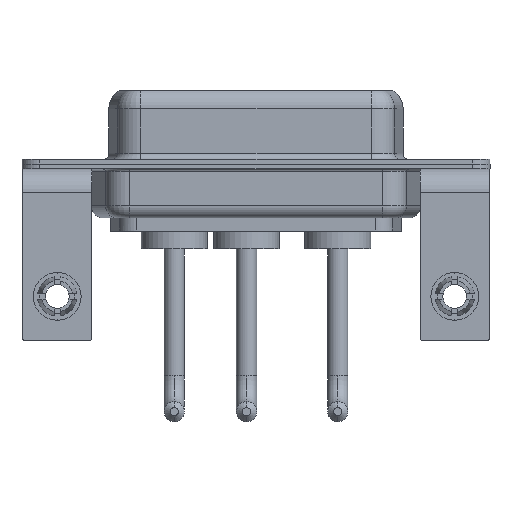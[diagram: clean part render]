
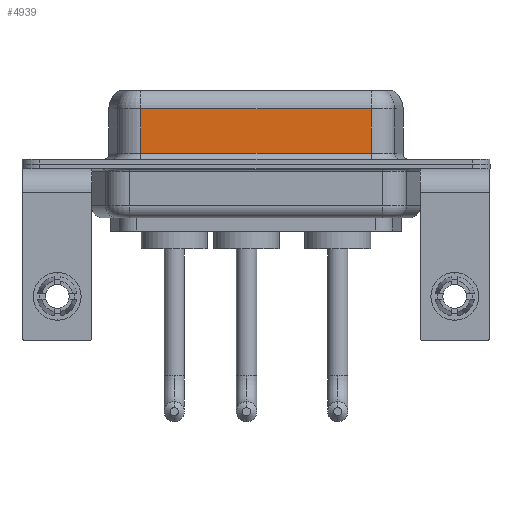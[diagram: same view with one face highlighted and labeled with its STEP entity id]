
A CAD part, front view. The second image highlights one B-rep face of the part: STEP entity #4939.
In plain terms, the highlighted planar face has unit normal (0, -1, 0).
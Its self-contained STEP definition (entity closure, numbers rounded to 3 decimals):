
#678 = DIRECTION ( 'NONE',  ( -1., 0., 0. ) ) ;
#1206 = DIRECTION ( 'NONE',  ( 0., 0., 1. ) ) ;
#1521 = ORIENTED_EDGE ( 'NONE', *, *, #10036, .T. ) ;
#1938 = LINE ( 'NONE', #8073, #7045 ) ;
#2019 = ORIENTED_EDGE ( 'NONE', *, *, #6612, .F. ) ;
#2343 = VECTOR ( 'NONE', #5146, 1000. ) ;
#2589 = PLANE ( 'NONE',  #15162 ) ;
#3071 = VERTEX_POINT ( 'NONE', #11148 ) ;
#3496 = VECTOR ( 'NONE', #678, 1000. ) ;
#3511 = CARTESIAN_POINT ( 'NONE',  ( 26.287, -3.95, 6.4 ) ) ;
#4939 = ADVANCED_FACE ( 'NONE', ( #13759 ), #2589, .F. ) ;
#5129 = EDGE_CURVE ( 'NONE', #3071, #7591, #12925, .T. ) ;
#5146 = DIRECTION ( 'NONE',  ( 0., 0., -1. ) ) ;
#6200 = ORIENTED_EDGE ( 'NONE', *, *, #11894, .T. ) ;
#6254 = DIRECTION ( 'NONE',  ( 1., 0., 0. ) ) ;
#6612 = EDGE_CURVE ( 'NONE', #15115, #10348, #1938, .T. ) ;
#6883 = VECTOR ( 'NONE', #6254, 1000. ) ;
#6936 = DIRECTION ( 'NONE',  ( 0., 0., -1. ) ) ;
#7045 = VECTOR ( 'NONE', #6936, 1000. ) ;
#7591 = VERTEX_POINT ( 'NONE', #14528 ) ;
#7631 = CARTESIAN_POINT ( 'NONE',  ( 26.287, -3.95, 0.9 ) ) ;
#7859 = LINE ( 'NONE', #12967, #3496 ) ;
#8073 = CARTESIAN_POINT ( 'NONE',  ( 26.287, -3.95, 6.4 ) ) ;
#9892 = DIRECTION ( 'NONE',  ( 0., 1., 0. ) ) ;
#10036 = EDGE_CURVE ( 'NONE', #7591, #10348, #10103, .T. ) ;
#10103 = LINE ( 'NONE', #7631, #6883 ) ;
#10130 = CARTESIAN_POINT ( 'NONE',  ( 7.013, -3.95, 6.4 ) ) ;
#10348 = VERTEX_POINT ( 'NONE', #13313 ) ;
#11148 = CARTESIAN_POINT ( 'NONE',  ( 7.013, -3.95, 4.65 ) ) ;
#11894 = EDGE_CURVE ( 'NONE', #15115, #3071, #7859, .T. ) ;
#12925 = LINE ( 'NONE', #10130, #2343 ) ;
#12967 = CARTESIAN_POINT ( 'NONE',  ( 26.287, -3.95, 4.65 ) ) ;
#13032 = ORIENTED_EDGE ( 'NONE', *, *, #5129, .T. ) ;
#13313 = CARTESIAN_POINT ( 'NONE',  ( 26.287, -3.95, 0.9 ) ) ;
#13759 = FACE_OUTER_BOUND ( 'NONE', #14324, .T. ) ;
#14324 = EDGE_LOOP ( 'NONE', ( #2019, #6200, #13032, #1521 ) ) ;
#14528 = CARTESIAN_POINT ( 'NONE',  ( 7.013, -3.95, 0.9 ) ) ;
#15084 = CARTESIAN_POINT ( 'NONE',  ( 26.287, -3.95, 4.65 ) ) ;
#15115 = VERTEX_POINT ( 'NONE', #15084 ) ;
#15162 = AXIS2_PLACEMENT_3D ( 'NONE', #3511, #9892, #1206 ) ;
